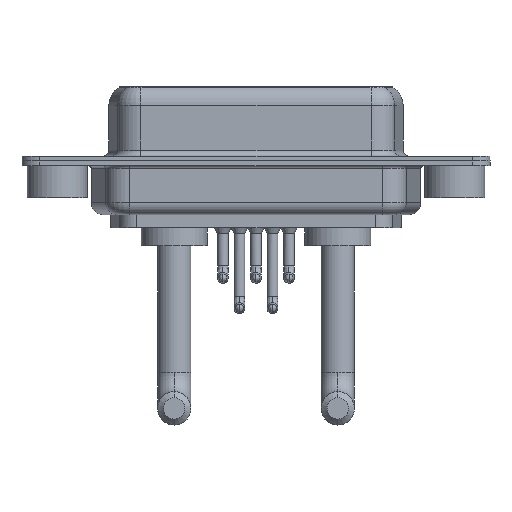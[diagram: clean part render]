
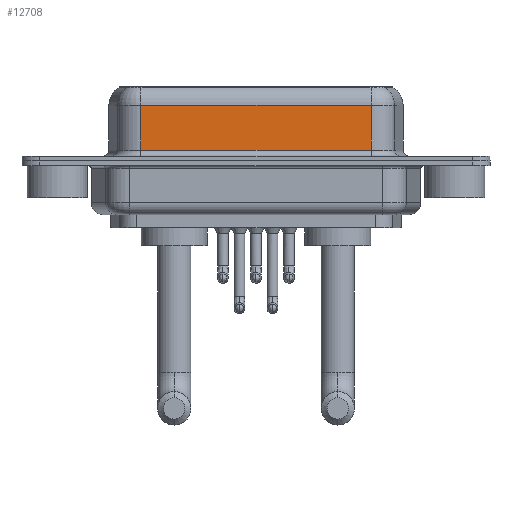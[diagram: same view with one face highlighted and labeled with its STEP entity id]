
A CAD part, front view. The second image highlights one B-rep face of the part: STEP entity #12708.
In plain terms, the highlighted planar face has unit normal (0, -1, 0).
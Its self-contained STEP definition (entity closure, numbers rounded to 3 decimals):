
#797 = EDGE_CURVE ( 'NONE', #3488, #12509, #8959, .T. ) ;
#824 = CARTESIAN_POINT ( 'NONE',  ( 26.287, -3.95, 6.4 ) ) ;
#1068 = CARTESIAN_POINT ( 'NONE',  ( 26.287, -3.95, 4.65 ) ) ;
#1713 = CARTESIAN_POINT ( 'NONE',  ( 26.287, -3.95, 4.65 ) ) ;
#1892 = VERTEX_POINT ( 'NONE', #13913 ) ;
#2096 = LINE ( 'NONE', #7231, #8147 ) ;
#2359 = CARTESIAN_POINT ( 'NONE',  ( 26.287, -3.95, 6.4 ) ) ;
#3053 = DIRECTION ( 'NONE',  ( 0., 0., 1. ) ) ;
#3389 = PLANE ( 'NONE',  #11129 ) ;
#3488 = VERTEX_POINT ( 'NONE', #1713 ) ;
#4035 = CARTESIAN_POINT ( 'NONE',  ( 7.013, -3.95, 0.9 ) ) ;
#4212 = DIRECTION ( 'NONE',  ( 1., 0., 0. ) ) ;
#4300 = EDGE_CURVE ( 'NONE', #14424, #12509, #12016, .T. ) ;
#5600 = DIRECTION ( 'NONE',  ( 0., 0., -1. ) ) ;
#6439 = VECTOR ( 'NONE', #4212, 1000. ) ;
#6554 = LINE ( 'NONE', #1068, #11465 ) ;
#7231 = CARTESIAN_POINT ( 'NONE',  ( 7.013, -3.95, 6.4 ) ) ;
#8147 = VECTOR ( 'NONE', #5600, 1000. ) ;
#8959 = LINE ( 'NONE', #2359, #15818 ) ;
#9980 = DIRECTION ( 'NONE',  ( 0., 1., 0. ) ) ;
#10160 = ORIENTED_EDGE ( 'NONE', *, *, #4300, .T. ) ;
#10414 = DIRECTION ( 'NONE',  ( -1., 0., 0. ) ) ;
#11073 = ORIENTED_EDGE ( 'NONE', *, *, #13087, .T. ) ;
#11129 = AXIS2_PLACEMENT_3D ( 'NONE', #824, #9980, #3053 ) ;
#11465 = VECTOR ( 'NONE', #10414, 1000. ) ;
#12016 = LINE ( 'NONE', #15954, #6439 ) ;
#12509 = VERTEX_POINT ( 'NONE', #15993 ) ;
#12708 = ADVANCED_FACE ( 'NONE', ( #15137 ), #3389, .F. ) ;
#13087 = EDGE_CURVE ( 'NONE', #1892, #14424, #2096, .T. ) ;
#13913 = CARTESIAN_POINT ( 'NONE',  ( 7.013, -3.95, 4.65 ) ) ;
#14201 = ORIENTED_EDGE ( 'NONE', *, *, #797, .F. ) ;
#14424 = VERTEX_POINT ( 'NONE', #4035 ) ;
#14462 = ORIENTED_EDGE ( 'NONE', *, *, #15417, .T. ) ;
#14687 = EDGE_LOOP ( 'NONE', ( #14201, #14462, #11073, #10160 ) ) ;
#15137 = FACE_OUTER_BOUND ( 'NONE', #14687, .T. ) ;
#15210 = DIRECTION ( 'NONE',  ( 0., 0., -1. ) ) ;
#15417 = EDGE_CURVE ( 'NONE', #3488, #1892, #6554, .T. ) ;
#15818 = VECTOR ( 'NONE', #15210, 1000. ) ;
#15954 = CARTESIAN_POINT ( 'NONE',  ( 26.287, -3.95, 0.9 ) ) ;
#15993 = CARTESIAN_POINT ( 'NONE',  ( 26.287, -3.95, 0.9 ) ) ;
